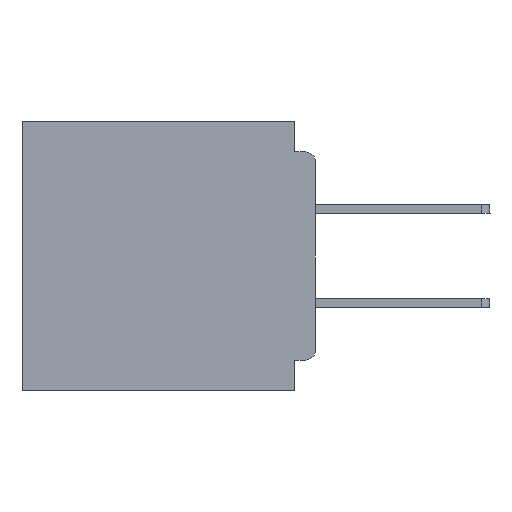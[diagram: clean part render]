
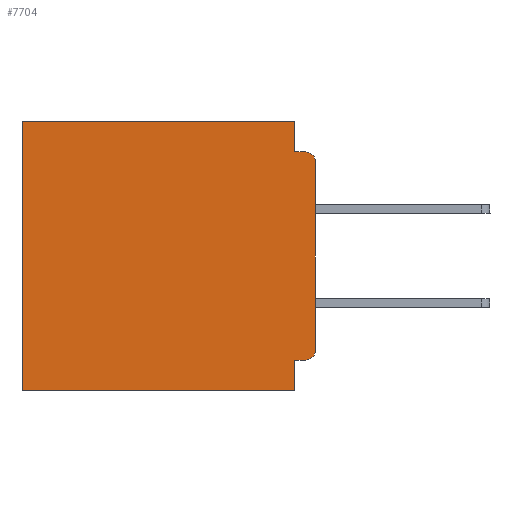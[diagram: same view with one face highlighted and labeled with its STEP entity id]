
A CAD part, left-side view. The second image highlights one B-rep face of the part: STEP entity #7704.
In plain terms, the highlighted planar face has unit normal (-1, 0, 0).
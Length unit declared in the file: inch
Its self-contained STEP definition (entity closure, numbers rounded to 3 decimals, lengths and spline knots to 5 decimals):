
#273 = VERTEX_POINT ( 'NONE', #62658 ) ;
#793 = CARTESIAN_POINT ( 'NONE',  ( 0.3, 0.015, -0.06 ) ) ;
#1339 = DIRECTION ( 'NONE',  ( 0., 0., -1. ) ) ;
#1350 = ORIENTED_EDGE ( 'NONE', *, *, #64326, .F. ) ;
#2122 = VERTEX_POINT ( 'NONE', #58281 ) ;
#2858 = VERTEX_POINT ( 'NONE', #52063 ) ;
#3582 = AXIS2_PLACEMENT_3D ( 'NONE', #41047, #11047, #46041 ) ;
#3794 = DIRECTION ( 'NONE',  ( 0., 0., -1. ) ) ;
#4633 = ORIENTED_EDGE ( 'NONE', *, *, #42976, .T. ) ;
#4930 = CARTESIAN_POINT ( 'NONE',  ( 0.3, 0., -0.045 ) ) ;
#5830 = DIRECTION ( 'NONE',  ( 0., 0., -1. ) ) ;
#6226 = ORIENTED_EDGE ( 'NONE', *, *, #39777, .T. ) ;
#7704 = ADVANCED_FACE ( 'NONE', ( #36871 ), #55528, .F. ) ;
#9012 = DIRECTION ( 'NONE',  ( -1., 0., 0. ) ) ;
#9186 = VERTEX_POINT ( 'NONE', #52801 ) ;
#9432 = EDGE_CURVE ( 'NONE', #273, #34875, #14726, .T. ) ;
#10346 = CARTESIAN_POINT ( 'NONE',  ( 0.3, 0.015, -0.355 ) ) ;
#11047 = DIRECTION ( 'NONE',  ( 1., 0., 0. ) ) ;
#13563 = DIRECTION ( 'NONE',  ( 0., 1., 0. ) ) ;
#13694 = CARTESIAN_POINT ( 'NONE',  ( 0.3, 0., -0.06 ) ) ;
#14580 = EDGE_CURVE ( 'NONE', #42544, #2858, #56641, .T. ) ;
#14726 = LINE ( 'NONE', #4930, #38204 ) ;
#15639 = EDGE_CURVE ( 'NONE', #56189, #39207, #36484, .T. ) ;
#16247 = CARTESIAN_POINT ( 'NONE',  ( 0.3, 0.031, -0.4 ) ) ;
#17785 = CARTESIAN_POINT ( 'NONE',  ( 0.3, 0., -0.355 ) ) ;
#18478 = CARTESIAN_POINT ( 'NONE',  ( 0.3, 0.015, -0.045 ) ) ;
#20004 = AXIS2_PLACEMENT_3D ( 'NONE', #793, #35869, #5830 ) ;
#20024 = LINE ( 'NONE', #27707, #46603 ) ;
#20279 = EDGE_CURVE ( 'NONE', #50864, #39207, #51086, .T. ) ;
#21292 = CARTESIAN_POINT ( 'NONE',  ( 0.3, 0., -0.4 ) ) ;
#21374 = EDGE_CURVE ( 'NONE', #32709, #9186, #33803, .T. ) ;
#24579 = EDGE_LOOP ( 'NONE', ( #36285, #4633, #29836, #1350, #61579, #6226, #50465, #61028, #34892, #53379 ) ) ;
#27707 = CARTESIAN_POINT ( 'NONE',  ( 0.3, 0.031, -0.4 ) ) ;
#27794 = DIRECTION ( 'NONE',  ( 0., 1., 0. ) ) ;
#29836 = ORIENTED_EDGE ( 'NONE', *, *, #9432, .F. ) ;
#30194 = VECTOR ( 'NONE', #58599, 39.37008 ) ;
#32345 = LINE ( 'NONE', #17785, #57203 ) ;
#32709 = VERTEX_POINT ( 'NONE', #40716 ) ;
#32751 = DIRECTION ( 'NONE',  ( 0., 0., -1. ) ) ;
#33803 = LINE ( 'NONE', #63114, #58613 ) ;
#34758 = CARTESIAN_POINT ( 'NONE',  ( 0.3, 0.437, -0.4 ) ) ;
#34875 = VERTEX_POINT ( 'NONE', #18478 ) ;
#34888 = VECTOR ( 'NONE', #1339, 39.37008 ) ;
#34892 = ORIENTED_EDGE ( 'NONE', *, *, #49155, .F. ) ;
#35869 = DIRECTION ( 'NONE',  ( -1., 0., 0. ) ) ;
#36285 = ORIENTED_EDGE ( 'NONE', *, *, #15639, .F. ) ;
#36484 = LINE ( 'NONE', #21292, #34888 ) ;
#36871 = FACE_OUTER_BOUND ( 'NONE', #24579, .T. ) ;
#38204 = VECTOR ( 'NONE', #54688, 39.37008 ) ;
#38942 = CARTESIAN_POINT ( 'NONE',  ( 0.3, 0., -0.4 ) ) ;
#39041 = CARTESIAN_POINT ( 'NONE',  ( 0.3, 0.015, -0.34 ) ) ;
#39207 = VERTEX_POINT ( 'NONE', #54550 ) ;
#39499 = VECTOR ( 'NONE', #3794, 39.37008 ) ;
#39777 = EDGE_CURVE ( 'NONE', #9186, #2858, #63470, .T. ) ;
#39787 = DIRECTION ( 'NONE',  ( 0., 0., -1. ) ) ;
#40716 = CARTESIAN_POINT ( 'NONE',  ( 0.3, 0.031, 0. ) ) ;
#41047 = CARTESIAN_POINT ( 'NONE',  ( 0.3, 0., -0.4 ) ) ;
#42544 = VERTEX_POINT ( 'NONE', #16247 ) ;
#42976 = EDGE_CURVE ( 'NONE', #56189, #34875, #52977, .T. ) ;
#44056 = DIRECTION ( 'NONE',  ( 0., 0., -1. ) ) ;
#46041 = DIRECTION ( 'NONE',  ( 0., 0., -1. ) ) ;
#46603 = VECTOR ( 'NONE', #32751, 39.37008 ) ;
#48027 = EDGE_CURVE ( 'NONE', #2122, #42544, #20024, .T. ) ;
#49155 = EDGE_CURVE ( 'NONE', #50864, #2122, #32345, .T. ) ;
#50362 = VECTOR ( 'NONE', #39787, 39.37008 ) ;
#50465 = ORIENTED_EDGE ( 'NONE', *, *, #14580, .F. ) ;
#50864 = VERTEX_POINT ( 'NONE', #10346 ) ;
#51086 = CIRCLE ( 'NONE', #55122, 0.015 ) ;
#52063 = CARTESIAN_POINT ( 'NONE',  ( 0.3, 0.437, -0.4 ) ) ;
#52686 = LINE ( 'NONE', #53382, #39499 ) ;
#52801 = CARTESIAN_POINT ( 'NONE',  ( 0.3, 0.437, 0. ) ) ;
#52977 = CIRCLE ( 'NONE', #20004, 0.015 ) ;
#53379 = ORIENTED_EDGE ( 'NONE', *, *, #20279, .T. ) ;
#53382 = CARTESIAN_POINT ( 'NONE',  ( 0.3, 0.031, 0. ) ) ;
#54550 = CARTESIAN_POINT ( 'NONE',  ( 0.3, 0., -0.34 ) ) ;
#54688 = DIRECTION ( 'NONE',  ( 0., -1., 0. ) ) ;
#55122 = AXIS2_PLACEMENT_3D ( 'NONE', #39041, #9012, #44056 ) ;
#55528 = PLANE ( 'NONE',  #3582 ) ;
#56189 = VERTEX_POINT ( 'NONE', #13694 ) ;
#56641 = LINE ( 'NONE', #38942, #30194 ) ;
#57203 = VECTOR ( 'NONE', #27794, 39.37008 ) ;
#58281 = CARTESIAN_POINT ( 'NONE',  ( 0.3, 0.031, -0.355 ) ) ;
#58599 = DIRECTION ( 'NONE',  ( 0., 1., 0. ) ) ;
#58613 = VECTOR ( 'NONE', #13563, 39.37008 ) ;
#61028 = ORIENTED_EDGE ( 'NONE', *, *, #48027, .F. ) ;
#61579 = ORIENTED_EDGE ( 'NONE', *, *, #21374, .T. ) ;
#62658 = CARTESIAN_POINT ( 'NONE',  ( 0.3, 0.031, -0.045 ) ) ;
#63114 = CARTESIAN_POINT ( 'NONE',  ( 0.3, 0., 0. ) ) ;
#63470 = LINE ( 'NONE', #34758, #50362 ) ;
#64326 = EDGE_CURVE ( 'NONE', #32709, #273, #52686, .T. ) ;
